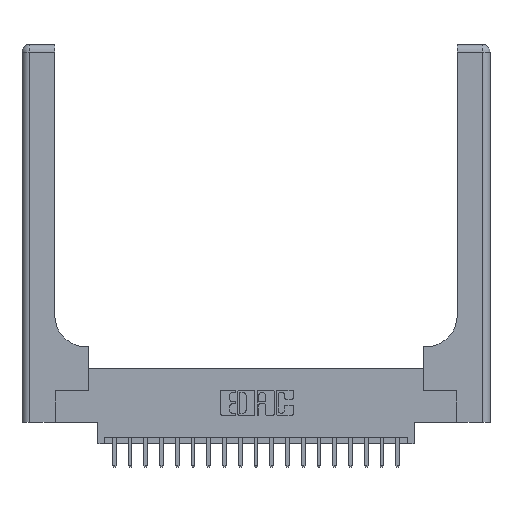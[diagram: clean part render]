
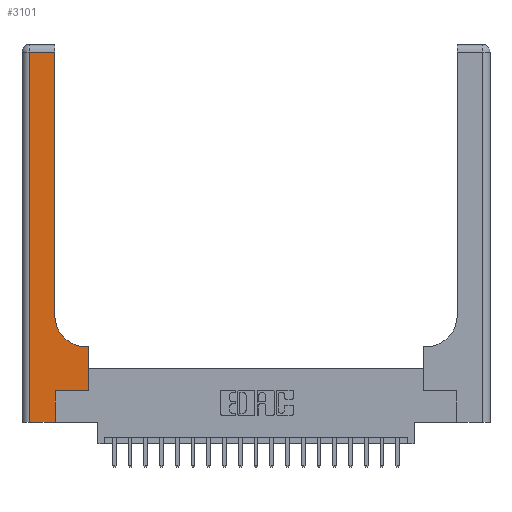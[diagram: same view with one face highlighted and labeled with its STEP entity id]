
A CAD part, top view. The second image highlights one B-rep face of the part: STEP entity #3101.
In plain terms, the highlighted planar face has unit normal (0, 0, 1).
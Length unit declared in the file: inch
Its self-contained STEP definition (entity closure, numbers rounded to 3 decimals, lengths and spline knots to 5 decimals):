
#24 = CARTESIAN_POINT ( 'NONE',  ( 0.51, 0.85, 0.37 ) ) ;
#39 = ORIENTED_EDGE ( 'NONE', *, *, #5757, .T. ) ;
#275 = VECTOR ( 'NONE', #6382, 39.37008 ) ;
#347 = LINE ( 'NONE', #8031, #8428 ) ;
#819 = CARTESIAN_POINT ( 'NONE',  ( 0.51, 0.6, 0.37 ) ) ;
#933 = LINE ( 'NONE', #12227, #18166 ) ;
#1281 = EDGE_CURVE ( 'NONE', #17880, #17476, #933, .T. ) ;
#1313 = CARTESIAN_POINT ( 'NONE',  ( 0.26, 2.94, 0.37 ) ) ;
#1585 = DIRECTION ( 'NONE',  ( 0., 1., 0. ) ) ;
#1618 = DIRECTION ( 'NONE',  ( 1., 0., 0. ) ) ;
#1709 = PLANE ( 'NONE',  #10974 ) ;
#1816 = VERTEX_POINT ( 'NONE', #10236 ) ;
#1820 = VECTOR ( 'NONE', #20609, 39.37008 ) ;
#2120 = CIRCLE ( 'NONE', #3951, 0.25 ) ;
#2533 = DIRECTION ( 'NONE',  ( 1., 0., 0. ) ) ;
#2616 = CARTESIAN_POINT ( 'NONE',  ( 0.528, 0.25, 0.37 ) ) ;
#2719 = ORIENTED_EDGE ( 'NONE', *, *, #16214, .T. ) ;
#2729 = VECTOR ( 'NONE', #13168, 39.37008 ) ;
#3101 = ADVANCED_FACE ( 'NONE', ( #20617 ), #1709, .F. ) ;
#3337 = DIRECTION ( 'NONE',  ( 0., 0., -1. ) ) ;
#3951 = AXIS2_PLACEMENT_3D ( 'NONE', #24, #11324, #1618 ) ;
#4075 = LINE ( 'NONE', #19313, #275 ) ;
#4084 = VERTEX_POINT ( 'NONE', #19076 ) ;
#4514 = ORIENTED_EDGE ( 'NONE', *, *, #5306, .T. ) ;
#4580 = LINE ( 'NONE', #13108, #8865 ) ;
#5158 = EDGE_CURVE ( 'NONE', #18194, #4084, #19013, .T. ) ;
#5306 = EDGE_CURVE ( 'NONE', #17476, #18194, #4075, .T. ) ;
#5581 = CARTESIAN_POINT ( 'NONE',  ( 0.06, 2.94, 0.37 ) ) ;
#5641 = EDGE_CURVE ( 'NONE', #4084, #1816, #14688, .T. ) ;
#5757 = EDGE_CURVE ( 'NONE', #1816, #15893, #4580, .T. ) ;
#6091 = VECTOR ( 'NONE', #1585, 39.37008 ) ;
#6134 = CARTESIAN_POINT ( 'NONE',  ( 0.265, 0., 0.37 ) ) ;
#6382 = DIRECTION ( 'NONE',  ( 0., 1., 0. ) ) ;
#7240 = ORIENTED_EDGE ( 'NONE', *, *, #5641, .T. ) ;
#7539 = LINE ( 'NONE', #8361, #2729 ) ;
#7600 = CARTESIAN_POINT ( 'NONE',  ( 0.26, 0.85, 0.37 ) ) ;
#7634 = CARTESIAN_POINT ( 'NONE',  ( 0.265, 0.25, 0.37 ) ) ;
#8031 = CARTESIAN_POINT ( 'NONE',  ( 0., 2.94, 0.37 ) ) ;
#8149 = CARTESIAN_POINT ( 'NONE',  ( 0., 3., 0.37 ) ) ;
#8361 = CARTESIAN_POINT ( 'NONE',  ( 0.26, 3., 0.37 ) ) ;
#8428 = VECTOR ( 'NONE', #12906, 39.37008 ) ;
#8430 = VERTEX_POINT ( 'NONE', #5581 ) ;
#8865 = VECTOR ( 'NONE', #14742, 39.37008 ) ;
#9284 = DIRECTION ( 'NONE',  ( 1., 0., 0. ) ) ;
#9912 = ORIENTED_EDGE ( 'NONE', *, *, #13466, .T. ) ;
#10236 = CARTESIAN_POINT ( 'NONE',  ( 0.528, 0.6, 0.37 ) ) ;
#10430 = LINE ( 'NONE', #18976, #1820 ) ;
#10974 = AXIS2_PLACEMENT_3D ( 'NONE', #8149, #3337, #14656 ) ;
#11324 = DIRECTION ( 'NONE',  ( 0., 0., -1. ) ) ;
#11673 = ORIENTED_EDGE ( 'NONE', *, *, #12003, .T. ) ;
#12003 = EDGE_CURVE ( 'NONE', #15893, #17432, #2120, .T. ) ;
#12053 = ORIENTED_EDGE ( 'NONE', *, *, #5158, .T. ) ;
#12227 = CARTESIAN_POINT ( 'NONE',  ( 0., 0., 0.37 ) ) ;
#12906 = DIRECTION ( 'NONE',  ( -1., 0., 0. ) ) ;
#13108 = CARTESIAN_POINT ( 'NONE',  ( 0.26, 0.6, 0.37 ) ) ;
#13168 = DIRECTION ( 'NONE',  ( 0., 1., 0. ) ) ;
#13466 = EDGE_CURVE ( 'NONE', #17432, #17504, #7539, .T. ) ;
#14163 = CARTESIAN_POINT ( 'NONE',  ( 0.06, 0., 0.37 ) ) ;
#14656 = DIRECTION ( 'NONE',  ( -1., 0., 0. ) ) ;
#14688 = LINE ( 'NONE', #2616, #6091 ) ;
#14742 = DIRECTION ( 'NONE',  ( -1., 0., 0. ) ) ;
#15792 = ORIENTED_EDGE ( 'NONE', *, *, #1281, .T. ) ;
#15807 = ORIENTED_EDGE ( 'NONE', *, *, #17861, .T. ) ;
#15893 = VERTEX_POINT ( 'NONE', #819 ) ;
#16214 = EDGE_CURVE ( 'NONE', #17504, #8430, #347, .T. ) ;
#17432 = VERTEX_POINT ( 'NONE', #7600 ) ;
#17476 = VERTEX_POINT ( 'NONE', #6134 ) ;
#17504 = VERTEX_POINT ( 'NONE', #1313 ) ;
#17861 = EDGE_CURVE ( 'NONE', #8430, #17880, #10430, .T. ) ;
#17880 = VERTEX_POINT ( 'NONE', #14163 ) ;
#18166 = VECTOR ( 'NONE', #2533, 39.37008 ) ;
#18192 = CARTESIAN_POINT ( 'NONE',  ( 0.265, 0.25, 0.37 ) ) ;
#18194 = VERTEX_POINT ( 'NONE', #18192 ) ;
#18500 = VECTOR ( 'NONE', #9284, 39.37008 ) ;
#18976 = CARTESIAN_POINT ( 'NONE',  ( 0.06, 3., 0.37 ) ) ;
#19013 = LINE ( 'NONE', #7634, #18500 ) ;
#19076 = CARTESIAN_POINT ( 'NONE',  ( 0.528, 0.25, 0.37 ) ) ;
#19203 = EDGE_LOOP ( 'NONE', ( #9912, #2719, #15807, #15792, #4514, #12053, #7240, #39, #11673 ) ) ;
#19313 = CARTESIAN_POINT ( 'NONE',  ( 0.265, 0., 0.37 ) ) ;
#20609 = DIRECTION ( 'NONE',  ( 0., -1., 0. ) ) ;
#20617 = FACE_OUTER_BOUND ( 'NONE', #19203, .T. ) ;
